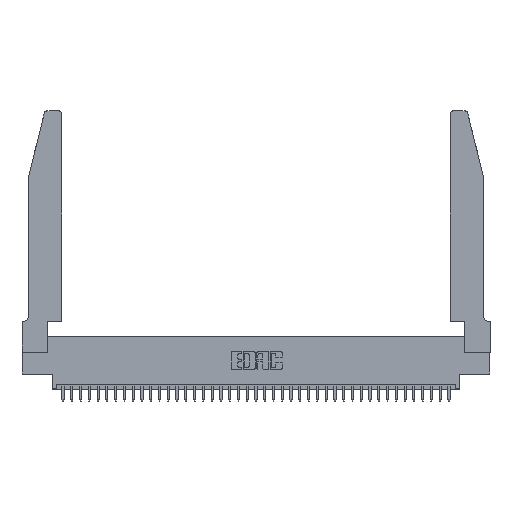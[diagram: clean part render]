
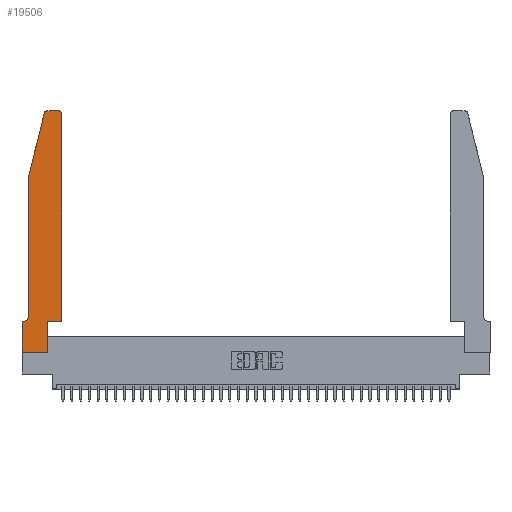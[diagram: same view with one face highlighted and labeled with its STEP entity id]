
A CAD part, top view. The second image highlights one B-rep face of the part: STEP entity #19506.
In plain terms, the highlighted planar face has unit normal (0, 0, 1).
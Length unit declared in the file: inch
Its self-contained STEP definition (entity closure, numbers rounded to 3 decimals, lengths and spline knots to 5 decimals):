
#365 = CARTESIAN_POINT ( 'NONE',  ( 0.4205, 2.75, 0.37 ) ) ;
#493 = CARTESIAN_POINT ( 'NONE',  ( 0.4505, 0.35, 0.37 ) ) ;
#1320 = DIRECTION ( 'NONE',  ( 1., 0., 0. ) ) ;
#1839 = ORIENTED_EDGE ( 'NONE', *, *, #33229, .T. ) ;
#2216 = AXIS2_PLACEMENT_3D ( 'NONE', #9982, #25528, #6978 ) ;
#2516 = DIRECTION ( 'NONE',  ( 0., -1., 0. ) ) ;
#2965 = EDGE_CURVE ( 'NONE', #21279, #23780, #20093, .T. ) ;
#2992 = DIRECTION ( 'NONE',  ( 1., 0., 0. ) ) ;
#3176 = EDGE_CURVE ( 'NONE', #37328, #16672, #14794, .T. ) ;
#3876 = PLANE ( 'NONE',  #2216 ) ;
#4175 = ORIENTED_EDGE ( 'NONE', *, *, #32545, .T. ) ;
#4525 = EDGE_CURVE ( 'NONE', #34246, #19390, #8404, .T. ) ;
#5292 = LINE ( 'NONE', #27131, #37059 ) ;
#5624 = VECTOR ( 'NONE', #12553, 39.37008 ) ;
#6059 = CARTESIAN_POINT ( 'NONE',  ( 0.0055, 0.35, 0.37 ) ) ;
#6978 = DIRECTION ( 'NONE',  ( 1., 0., 0. ) ) ;
#7117 = CARTESIAN_POINT ( 'NONE',  ( 0.0755, 2., 0.37 ) ) ;
#8404 = CIRCLE ( 'NONE', #22362, 0.03 ) ;
#9198 = ORIENTED_EDGE ( 'NONE', *, *, #35929, .T. ) ;
#9394 = VERTEX_POINT ( 'NONE', #38092 ) ;
#9982 = CARTESIAN_POINT ( 'NONE',  ( 0., 0.35, 0.37 ) ) ;
#10247 = CARTESIAN_POINT ( 'NONE',  ( 0.2605, 2.75, 0.37 ) ) ;
#10498 = LINE ( 'NONE', #20426, #17713 ) ;
#11092 = CARTESIAN_POINT ( 'NONE',  ( 0.4505, 0.35, 0.37 ) ) ;
#11382 = CARTESIAN_POINT ( 'NONE',  ( 0.2865, 0.35, 0.37 ) ) ;
#11456 = LINE ( 'NONE', #29468, #26956 ) ;
#12010 = LINE ( 'NONE', #493, #27499 ) ;
#12385 = VERTEX_POINT ( 'NONE', #37341 ) ;
#12553 = DIRECTION ( 'NONE',  ( -0.239, -0.971, 0. ) ) ;
#13342 = DIRECTION ( 'NONE',  ( -1., 0., 0. ) ) ;
#14078 = CARTESIAN_POINT ( 'NONE',  ( 0.4205, 2.72, 0.37 ) ) ;
#14327 = FACE_OUTER_BOUND ( 'NONE', #26905, .T. ) ;
#14794 = LINE ( 'NONE', #15404, #5624 ) ;
#14972 = VECTOR ( 'NONE', #13342, 39.37008 ) ;
#15404 = CARTESIAN_POINT ( 'NONE',  ( 0.0755, 2., 0.37 ) ) ;
#15935 = LINE ( 'NONE', #10247, #14972 ) ;
#16057 = ORIENTED_EDGE ( 'NONE', *, *, #34651, .T. ) ;
#16099 = ORIENTED_EDGE ( 'NONE', *, *, #3176, .T. ) ;
#16569 = EDGE_CURVE ( 'NONE', #30528, #9394, #22318, .T. ) ;
#16672 = VERTEX_POINT ( 'NONE', #7117 ) ;
#16842 = CARTESIAN_POINT ( 'NONE',  ( 0.2865, 0., 0.37 ) ) ;
#17147 = DIRECTION ( 'NONE',  ( 1., 0., 0. ) ) ;
#17279 = DIRECTION ( 'NONE',  ( 1., 0., 0. ) ) ;
#17698 = ORIENTED_EDGE ( 'NONE', *, *, #2965, .T. ) ;
#17713 = VECTOR ( 'NONE', #23566, 39.37008 ) ;
#18125 = CARTESIAN_POINT ( 'NONE',  ( 0.0055, 0.42, 0.37 ) ) ;
#18465 = ORIENTED_EDGE ( 'NONE', *, *, #38049, .T. ) ;
#19281 = DIRECTION ( 'NONE',  ( 0., 1., 0. ) ) ;
#19390 = VERTEX_POINT ( 'NONE', #365 ) ;
#19506 = ADVANCED_FACE ( 'NONE', ( #14327 ), #3876, .T. ) ;
#19886 = CARTESIAN_POINT ( 'NONE',  ( 0., 0., 0.37 ) ) ;
#20093 = LINE ( 'NONE', #32141, #28340 ) ;
#20426 = CARTESIAN_POINT ( 'NONE',  ( 0., 0., 0.37 ) ) ;
#20585 = VERTEX_POINT ( 'NONE', #28300 ) ;
#21258 = DIRECTION ( 'NONE',  ( -1., 0., 0. ) ) ;
#21279 = VERTEX_POINT ( 'NONE', #19886 ) ;
#21400 = VERTEX_POINT ( 'NONE', #11092 ) ;
#21489 = DIRECTION ( 'NONE',  ( 0., 0., 1. ) ) ;
#21694 = CARTESIAN_POINT ( 'NONE',  ( 0.4505, 2.72, 0.37 ) ) ;
#22212 = CARTESIAN_POINT ( 'NONE',  ( 0.2865, 0.35, 0.37 ) ) ;
#22318 = LINE ( 'NONE', #33837, #28597 ) ;
#22362 = AXIS2_PLACEMENT_3D ( 'NONE', #14078, #35583, #17147 ) ;
#22435 = ORIENTED_EDGE ( 'NONE', *, *, #35655, .T. ) ;
#23566 = DIRECTION ( 'NONE',  ( 0., -1., 0. ) ) ;
#23780 = VERTEX_POINT ( 'NONE', #16842 ) ;
#24729 = VECTOR ( 'NONE', #35871, 39.37008 ) ;
#25480 = CIRCLE ( 'NONE', #34397, 0.03 ) ;
#25528 = DIRECTION ( 'NONE',  ( 0., 0., 1. ) ) ;
#26227 = EDGE_CURVE ( 'NONE', #23780, #34892, #32868, .T. ) ;
#26253 = ORIENTED_EDGE ( 'NONE', *, *, #38304, .T. ) ;
#26905 = EDGE_LOOP ( 'NONE', ( #22435, #26253, #16099, #9198, #16057, #30647, #18465, #17698, #33961, #1839, #4175, #34742 ) ) ;
#26956 = VECTOR ( 'NONE', #17279, 39.37008 ) ;
#27131 = CARTESIAN_POINT ( 'NONE',  ( 0.0755, 2., 0.37 ) ) ;
#27499 = VECTOR ( 'NONE', #19281, 39.37008 ) ;
#28300 = CARTESIAN_POINT ( 'NONE',  ( 0.284, 2.75, 0.37 ) ) ;
#28340 = VECTOR ( 'NONE', #1320, 39.37008 ) ;
#28597 = VECTOR ( 'NONE', #36870, 39.37008 ) ;
#29468 = CARTESIAN_POINT ( 'NONE',  ( 0.4505, 0.35, 0.37 ) ) ;
#30528 = VERTEX_POINT ( 'NONE', #6059 ) ;
#30647 = ORIENTED_EDGE ( 'NONE', *, *, #16569, .T. ) ;
#32141 = CARTESIAN_POINT ( 'NONE',  ( 0., 0., 0.37 ) ) ;
#32545 = EDGE_CURVE ( 'NONE', #21400, #34246, #12010, .T. ) ;
#32868 = LINE ( 'NONE', #11382, #24729 ) ;
#33229 = EDGE_CURVE ( 'NONE', #34892, #21400, #11456, .T. ) ;
#33837 = CARTESIAN_POINT ( 'NONE',  ( 0.0755, 0.35, 0.37 ) ) ;
#33961 = ORIENTED_EDGE ( 'NONE', *, *, #26227, .T. ) ;
#34246 = VERTEX_POINT ( 'NONE', #21694 ) ;
#34331 = CARTESIAN_POINT ( 'NONE',  ( 0.25487, 2.72718, 0.37 ) ) ;
#34397 = AXIS2_PLACEMENT_3D ( 'NONE', #39789, #21489, #2992 ) ;
#34581 = AXIS2_PLACEMENT_3D ( 'NONE', #18125, #39567, #21258 ) ;
#34651 = EDGE_CURVE ( 'NONE', #12385, #30528, #38214, .T. ) ;
#34742 = ORIENTED_EDGE ( 'NONE', *, *, #4525, .T. ) ;
#34892 = VERTEX_POINT ( 'NONE', #22212 ) ;
#35583 = DIRECTION ( 'NONE',  ( 0., 0., 1. ) ) ;
#35655 = EDGE_CURVE ( 'NONE', #19390, #20585, #15935, .T. ) ;
#35871 = DIRECTION ( 'NONE',  ( 0., 1., 0. ) ) ;
#35929 = EDGE_CURVE ( 'NONE', #16672, #12385, #5292, .T. ) ;
#36870 = DIRECTION ( 'NONE',  ( -1., 0., 0. ) ) ;
#37059 = VECTOR ( 'NONE', #2516, 39.37008 ) ;
#37328 = VERTEX_POINT ( 'NONE', #34331 ) ;
#37341 = CARTESIAN_POINT ( 'NONE',  ( 0.0755, 0.42, 0.37 ) ) ;
#38049 = EDGE_CURVE ( 'NONE', #9394, #21279, #10498, .T. ) ;
#38092 = CARTESIAN_POINT ( 'NONE',  ( 0., 0.35, 0.37 ) ) ;
#38214 = CIRCLE ( 'NONE', #34581, 0.07 ) ;
#38304 = EDGE_CURVE ( 'NONE', #20585, #37328, #25480, .T. ) ;
#39567 = DIRECTION ( 'NONE',  ( 0., 0., -1. ) ) ;
#39789 = CARTESIAN_POINT ( 'NONE',  ( 0.284, 2.72, 0.37 ) ) ;
